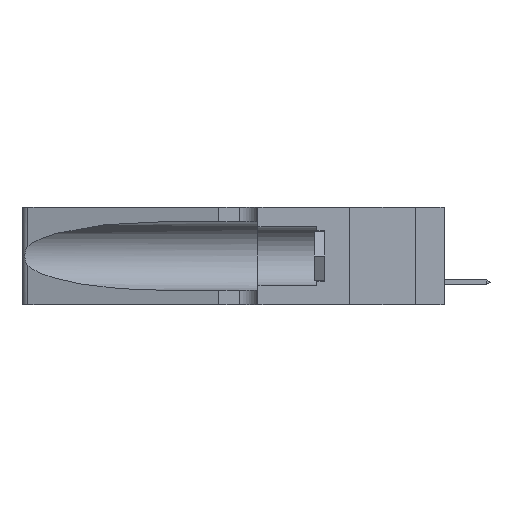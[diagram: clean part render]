
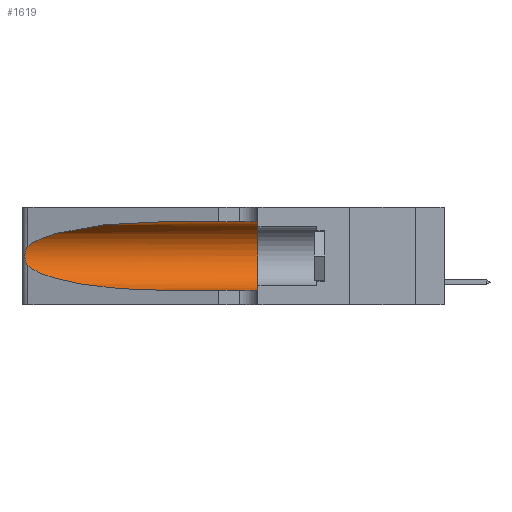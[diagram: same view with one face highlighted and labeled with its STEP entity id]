
A CAD part, left-side view. The second image highlights one B-rep face of the part: STEP entity #1619.
In plain terms, the highlighted cylindrical face has radius 3.308 mm (diameter 6.617 mm), a partial arc.
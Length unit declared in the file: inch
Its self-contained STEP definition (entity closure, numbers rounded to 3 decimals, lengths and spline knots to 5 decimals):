
#245 = EDGE_LOOP ( 'NONE', ( #27220, #19528, #28557, #9025, #4236, #12435 ) ) ;
#842 = VECTOR ( 'NONE', #23349, 39.37008 ) ;
#1239 = CARTESIAN_POINT ( 'NONE',  ( 0.1305, 1.61858, 0.05475 ) ) ;
#1489 = VERTEX_POINT ( 'NONE', #19059 ) ;
#1496 = B_SPLINE_CURVE_WITH_KNOTS ( 'NONE', 3,
 ( #13339, #24501, #11002, #28819, #4302, #4398, #15687, #13439, #9020, #28916, #15397, #11183, #6728, #17748 ),
 .UNSPECIFIED., .F., .F.,
 ( 4, 2, 2, 2, 2, 2, 4 ),
 ( 0., 0.00027, 0.00053, 0.00107, 0.0016, 0.00187, 0.00214 ),
 .UNSPECIFIED. ) ;
#1619 = ADVANCED_FACE ( 'NONE', ( #28709 ), #9406, .F. ) ;
#1903 = CARTESIAN_POINT ( 'NONE',  ( 0.18966, 0.96281, 0.31525 ) ) ;
#1984 = AXIS2_PLACEMENT_3D ( 'NONE', #18664, #16513, #5299 ) ;
#2074 = EDGE_CURVE ( 'NONE', #18788, #9335, #5677, .T. ) ;
#3945 = LINE ( 'NONE', #28293, #15881 ) ;
#4236 = ORIENTED_EDGE ( 'NONE', *, *, #16567, .F. ) ;
#4302 = CARTESIAN_POINT ( 'NONE',  ( 0.25854, 1.2359, 0.20912 ) ) ;
#4398 = CARTESIAN_POINT ( 'NONE',  ( 0.26018, 1.23835, 0.19895 ) ) ;
#4537 = EDGE_CURVE ( 'NONE', #1489, #15170, #3945, .T. ) ;
#4572 = CIRCLE ( 'NONE', #1984, 0.13025 ) ;
#5299 = DIRECTION ( 'NONE',  ( 0., 0., 1. ) ) ;
#5677 =( BOUNDED_CURVE ( )  B_SPLINE_CURVE ( 3, ( #11193, #22469, #13151, #13255 ),
 .UNSPECIFIED., .F., .F. ) 
 B_SPLINE_CURVE_WITH_KNOTS ( ( 4, 4 ),
 ( 3.44316, 4.71239 ),
 .UNSPECIFIED. ) 
 CURVE ( )  GEOMETRIC_REPRESENTATION_ITEM ( )  RATIONAL_B_SPLINE_CURVE ( ( 1., 0.87, 0.87, 1. ) ) 
 REPRESENTATION_ITEM ( '' )  );
#6728 = CARTESIAN_POINT ( 'NONE',  ( 0.25555, 1.22993, 0.14849 ) ) ;
#8416 = CARTESIAN_POINT ( 'NONE',  ( 0.2373, 1.15595, 0.28018 ) ) ;
#9020 = CARTESIAN_POINT ( 'NONE',  ( 0.26017, 1.23833, 0.17102 ) ) ;
#9025 = ORIENTED_EDGE ( 'NONE', *, *, #21600, .T. ) ;
#9284 = EDGE_CURVE ( 'NONE', #12664, #18788, #1496, .T. ) ;
#9335 = VERTEX_POINT ( 'NONE', #26841 ) ;
#9406 = CYLINDRICAL_SURFACE ( 'NONE', #13727, 0.13025 ) ;
#10139 = CARTESIAN_POINT ( 'NONE',  ( 0.25487, 1.22718, 0.22369 ) ) ;
#11002 = CARTESIAN_POINT ( 'NONE',  ( 0.25639, 1.23184, 0.21858 ) ) ;
#11183 = CARTESIAN_POINT ( 'NONE',  ( 0.25639, 1.23186, 0.15144 ) ) ;
#11193 = CARTESIAN_POINT ( 'NONE',  ( 0.25487, 1.22718, 0.14631 ) ) ;
#12435 = ORIENTED_EDGE ( 'NONE', *, *, #4537, .F. ) ;
#12664 = VERTEX_POINT ( 'NONE', #10139 ) ;
#12849 = CARTESIAN_POINT ( 'NONE',  ( 0.1305, 1.61858, 0.185 ) ) ;
#13151 = CARTESIAN_POINT ( 'NONE',  ( 0.18966, 0.96281, 0.05475 ) ) ;
#13255 = CARTESIAN_POINT ( 'NONE',  ( 0.1305, 0.72297, 0.05475 ) ) ;
#13339 = CARTESIAN_POINT ( 'NONE',  ( 0.25487, 1.22718, 0.22369 ) ) ;
#13439 = CARTESIAN_POINT ( 'NONE',  ( 0.26075, 1.23896, 0.178 ) ) ;
#13727 = AXIS2_PLACEMENT_3D ( 'NONE', #12849, #17143, #16853 ) ;
#15170 = VERTEX_POINT ( 'NONE', #28497 ) ;
#15397 = CARTESIAN_POINT ( 'NONE',  ( 0.25789, 1.23486, 0.15765 ) ) ;
#15687 = CARTESIAN_POINT ( 'NONE',  ( 0.26075, 1.23896, 0.19203 ) ) ;
#15881 = VECTOR ( 'NONE', #19563, 39.37008 ) ;
#16513 = DIRECTION ( 'NONE',  ( 0., 1., 0. ) ) ;
#16567 = EDGE_CURVE ( 'NONE', #15170, #25990, #4572, .T. ) ;
#16853 = DIRECTION ( 'NONE',  ( 0., 0., -1. ) ) ;
#17143 = DIRECTION ( 'NONE',  ( 0., -1., 0. ) ) ;
#17748 = CARTESIAN_POINT ( 'NONE',  ( 0.25487, 1.22718, 0.14631 ) ) ;
#18664 = CARTESIAN_POINT ( 'NONE',  ( 0.1305, 0.35, 0.185 ) ) ;
#18788 = VERTEX_POINT ( 'NONE', #22583 ) ;
#19059 = CARTESIAN_POINT ( 'NONE',  ( 0.1305, 0.72297, 0.31525 ) ) ;
#19528 = ORIENTED_EDGE ( 'NONE', *, *, #9284, .T. ) ;
#19563 = DIRECTION ( 'NONE',  ( 0., -1., 0. ) ) ;
#20243 =( BOUNDED_CURVE ( )  B_SPLINE_CURVE ( 3, ( #28421, #1903, #8416, #26355 ),
 .UNSPECIFIED., .F., .F. ) 
 B_SPLINE_CURVE_WITH_KNOTS ( ( 4, 4 ),
 ( 1.5708, 2.84003 ),
 .UNSPECIFIED. ) 
 CURVE ( )  GEOMETRIC_REPRESENTATION_ITEM ( )  RATIONAL_B_SPLINE_CURVE ( ( 1., 0.87, 0.87, 1. ) ) 
 REPRESENTATION_ITEM ( '' )  );
#20857 = EDGE_CURVE ( 'NONE', #1489, #12664, #20243, .T. ) ;
#21600 = EDGE_CURVE ( 'NONE', #9335, #25990, #24751, .T. ) ;
#22469 = CARTESIAN_POINT ( 'NONE',  ( 0.2373, 1.15595, 0.08982 ) ) ;
#22583 = CARTESIAN_POINT ( 'NONE',  ( 0.25487, 1.22718, 0.14631 ) ) ;
#23349 = DIRECTION ( 'NONE',  ( 0., -1., 0. ) ) ;
#24501 = CARTESIAN_POINT ( 'NONE',  ( 0.25555, 1.22994, 0.2215 ) ) ;
#24751 = LINE ( 'NONE', #1239, #842 ) ;
#25990 = VERTEX_POINT ( 'NONE', #27455 ) ;
#26355 = CARTESIAN_POINT ( 'NONE',  ( 0.25487, 1.22718, 0.22369 ) ) ;
#26841 = CARTESIAN_POINT ( 'NONE',  ( 0.1305, 0.72297, 0.05475 ) ) ;
#27220 = ORIENTED_EDGE ( 'NONE', *, *, #20857, .T. ) ;
#27455 = CARTESIAN_POINT ( 'NONE',  ( 0.1305, 0.35, 0.05475 ) ) ;
#28293 = CARTESIAN_POINT ( 'NONE',  ( 0.1305, 1.61858, 0.31525 ) ) ;
#28421 = CARTESIAN_POINT ( 'NONE',  ( 0.1305, 0.72297, 0.31525 ) ) ;
#28497 = CARTESIAN_POINT ( 'NONE',  ( 0.1305, 0.35, 0.31525 ) ) ;
#28557 = ORIENTED_EDGE ( 'NONE', *, *, #2074, .T. ) ;
#28709 = FACE_OUTER_BOUND ( 'NONE', #245, .T. ) ;
#28819 = CARTESIAN_POINT ( 'NONE',  ( 0.25787, 1.23484, 0.2124 ) ) ;
#28916 = CARTESIAN_POINT ( 'NONE',  ( 0.25856, 1.23593, 0.16098 ) ) ;
